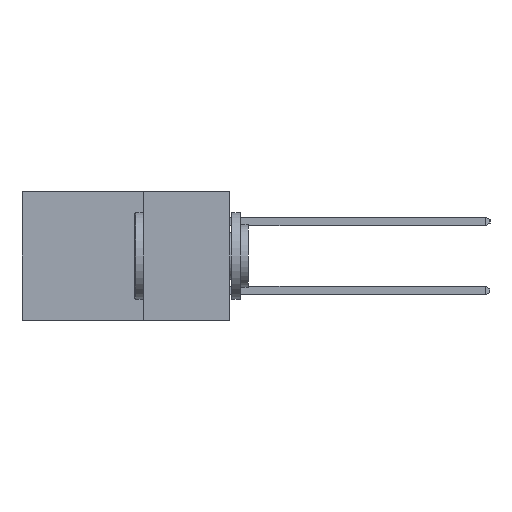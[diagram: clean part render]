
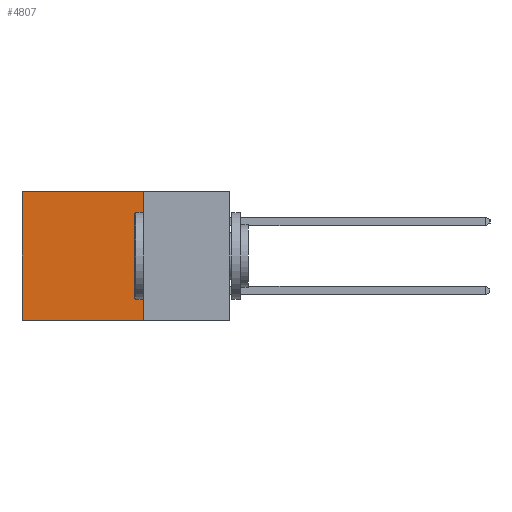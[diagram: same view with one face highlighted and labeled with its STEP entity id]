
A CAD part, left-side view. The second image highlights one B-rep face of the part: STEP entity #4807.
In plain terms, the highlighted planar face has unit normal (-1, 0, 0).
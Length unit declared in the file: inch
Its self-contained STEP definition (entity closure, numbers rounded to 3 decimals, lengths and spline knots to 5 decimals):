
#296 = CARTESIAN_POINT ( 'NONE',  ( 0.298, 0.25, -0.37 ) ) ;
#484 = LINE ( 'NONE', #12783, #12069 ) ;
#1005 = CARTESIAN_POINT ( 'NONE',  ( 0.298, 0.25, 0. ) ) ;
#1233 = PLANE ( 'NONE',  #7574 ) ;
#2018 = EDGE_CURVE ( 'NONE', #14423, #5466, #8580, .T. ) ;
#2658 = CARTESIAN_POINT ( 'NONE',  ( 0.298, 0.6, -0.37 ) ) ;
#3377 = DIRECTION ( 'NONE',  ( 0., 1., 0. ) ) ;
#3484 = ORIENTED_EDGE ( 'NONE', *, *, #2018, .T. ) ;
#4127 = DIRECTION ( 'NONE',  ( 0., 0., -1. ) ) ;
#4299 = VERTEX_POINT ( 'NONE', #8587 ) ;
#4473 = DIRECTION ( 'NONE',  ( 1., 0., 0. ) ) ;
#4610 = ORIENTED_EDGE ( 'NONE', *, *, #11571, .T. ) ;
#4807 = ADVANCED_FACE ( 'NONE', ( #8891 ), #1233, .F. ) ;
#5181 = CARTESIAN_POINT ( 'NONE',  ( 0.298, 0.25, 0. ) ) ;
#5466 = VERTEX_POINT ( 'NONE', #12340 ) ;
#5621 = VECTOR ( 'NONE', #4127, 39.37008 ) ;
#6431 = DIRECTION ( 'NONE',  ( 0., 1., 0. ) ) ;
#6773 = ORIENTED_EDGE ( 'NONE', *, *, #14752, .F. ) ;
#7574 = AXIS2_PLACEMENT_3D ( 'NONE', #1005, #4473, #13770 ) ;
#8569 = LINE ( 'NONE', #296, #10828 ) ;
#8580 = LINE ( 'NONE', #5181, #11169 ) ;
#8587 = CARTESIAN_POINT ( 'NONE',  ( 0.298, 0.25, -0.37 ) ) ;
#8891 = FACE_OUTER_BOUND ( 'NONE', #12450, .T. ) ;
#9656 = CARTESIAN_POINT ( 'NONE',  ( 0.298, 0.6, 0. ) ) ;
#9784 = ORIENTED_EDGE ( 'NONE', *, *, #11644, .F. ) ;
#9999 = VERTEX_POINT ( 'NONE', #2658 ) ;
#10828 = VECTOR ( 'NONE', #6431, 39.37008 ) ;
#11169 = VECTOR ( 'NONE', #3377, 39.37008 ) ;
#11571 = EDGE_CURVE ( 'NONE', #5466, #9999, #14490, .T. ) ;
#11644 = EDGE_CURVE ( 'NONE', #4299, #9999, #8569, .T. ) ;
#12069 = VECTOR ( 'NONE', #13938, 39.37008 ) ;
#12340 = CARTESIAN_POINT ( 'NONE',  ( 0.298, 0.6, 0. ) ) ;
#12450 = EDGE_LOOP ( 'NONE', ( #4610, #9784, #6773, #3484 ) ) ;
#12783 = CARTESIAN_POINT ( 'NONE',  ( 0.298, 0.25, 0. ) ) ;
#13661 = CARTESIAN_POINT ( 'NONE',  ( 0.298, 0.25, 0. ) ) ;
#13770 = DIRECTION ( 'NONE',  ( 0., 0., -1. ) ) ;
#13938 = DIRECTION ( 'NONE',  ( 0., 0., -1. ) ) ;
#14423 = VERTEX_POINT ( 'NONE', #13661 ) ;
#14490 = LINE ( 'NONE', #9656, #5621 ) ;
#14752 = EDGE_CURVE ( 'NONE', #14423, #4299, #484, .T. ) ;
